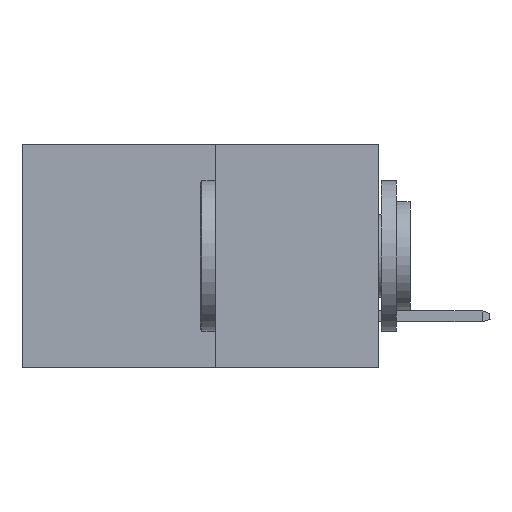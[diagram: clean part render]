
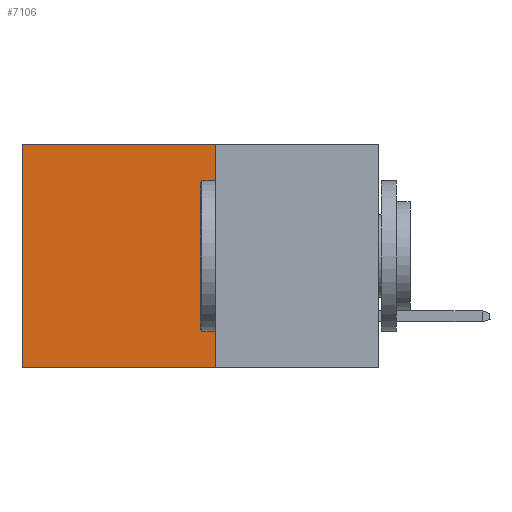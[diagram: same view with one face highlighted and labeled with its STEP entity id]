
A CAD part, left-side view. The second image highlights one B-rep face of the part: STEP entity #7106.
In plain terms, the highlighted planar face has unit normal (-1, 0, 0).
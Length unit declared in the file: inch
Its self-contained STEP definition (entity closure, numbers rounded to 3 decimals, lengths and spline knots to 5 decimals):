
#373 = EDGE_CURVE ( 'NONE', #19284, #6738, #26822, .T. ) ;
#1448 = LINE ( 'NONE', #2333, #7047 ) ;
#2199 = FACE_OUTER_BOUND ( 'NONE', #22776, .T. ) ;
#2333 = CARTESIAN_POINT ( 'NONE',  ( 0.277, 0.27, -0.37 ) ) ;
#3307 = DIRECTION ( 'NONE',  ( 0., 1., 0. ) ) ;
#4616 = PLANE ( 'NONE',  #26352 ) ;
#6585 = CARTESIAN_POINT ( 'NONE',  ( 0.277, 0.59, 0. ) ) ;
#6738 = VERTEX_POINT ( 'NONE', #17717 ) ;
#7008 = VERTEX_POINT ( 'NONE', #18783 ) ;
#7022 = DIRECTION ( 'NONE',  ( 1., 0., 0. ) ) ;
#7047 = VECTOR ( 'NONE', #21668, 39.37008 ) ;
#7106 = ADVANCED_FACE ( 'NONE', ( #2199 ), #4616, .F. ) ;
#7119 = EDGE_CURVE ( 'NONE', #7008, #16561, #1448, .T. ) ;
#7534 = VECTOR ( 'NONE', #23145, 39.37008 ) ;
#11005 = EDGE_CURVE ( 'NONE', #16561, #6738, #27082, .T. ) ;
#11065 = DIRECTION ( 'NONE',  ( 0., 1., 0. ) ) ;
#13607 = LINE ( 'NONE', #24956, #19287 ) ;
#16561 = VERTEX_POINT ( 'NONE', #20124 ) ;
#16833 = ORIENTED_EDGE ( 'NONE', *, *, #11005, .F. ) ;
#17717 = CARTESIAN_POINT ( 'NONE',  ( 0.277, 0.59, -0.37 ) ) ;
#17941 = ORIENTED_EDGE ( 'NONE', *, *, #373, .T. ) ;
#18783 = CARTESIAN_POINT ( 'NONE',  ( 0.277, 0.27, 0. ) ) ;
#19082 = CARTESIAN_POINT ( 'NONE',  ( 0.277, 0.59, -0.37 ) ) ;
#19090 = CARTESIAN_POINT ( 'NONE',  ( 0.277, 0.27, -0.37 ) ) ;
#19284 = VERTEX_POINT ( 'NONE', #6585 ) ;
#19287 = VECTOR ( 'NONE', #3307, 39.37008 ) ;
#20124 = CARTESIAN_POINT ( 'NONE',  ( 0.277, 0.27, -0.37 ) ) ;
#20704 = VECTOR ( 'NONE', #11065, 39.37008 ) ;
#20723 = CARTESIAN_POINT ( 'NONE',  ( 0.277, 0.27, -0.37 ) ) ;
#21487 = ORIENTED_EDGE ( 'NONE', *, *, #7119, .F. ) ;
#21668 = DIRECTION ( 'NONE',  ( 0., 0., -1. ) ) ;
#22776 = EDGE_LOOP ( 'NONE', ( #17941, #16833, #21487, #25331 ) ) ;
#23145 = DIRECTION ( 'NONE',  ( 0., 0., -1. ) ) ;
#23975 = DIRECTION ( 'NONE',  ( 0., 0., -1. ) ) ;
#24956 = CARTESIAN_POINT ( 'NONE',  ( 0.277, 0.27, 0. ) ) ;
#25331 = ORIENTED_EDGE ( 'NONE', *, *, #30317, .T. ) ;
#26352 = AXIS2_PLACEMENT_3D ( 'NONE', #19090, #7022, #23975 ) ;
#26822 = LINE ( 'NONE', #19082, #7534 ) ;
#27082 = LINE ( 'NONE', #20723, #20704 ) ;
#30317 = EDGE_CURVE ( 'NONE', #7008, #19284, #13607, .T. ) ;
